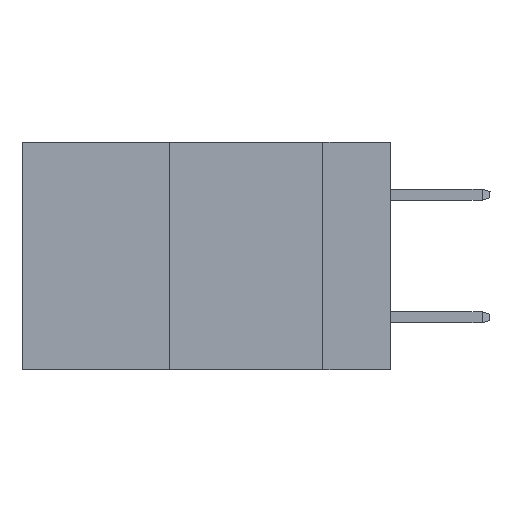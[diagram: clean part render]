
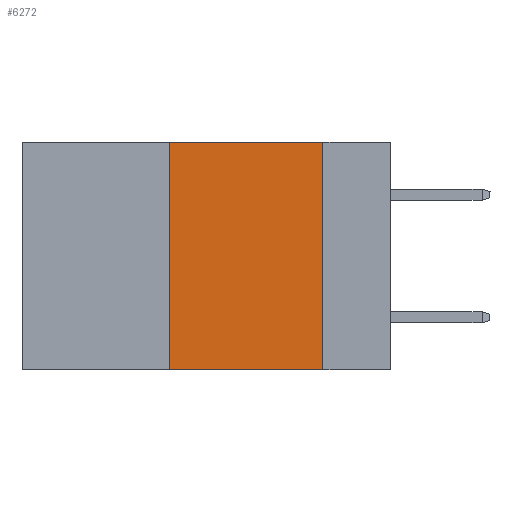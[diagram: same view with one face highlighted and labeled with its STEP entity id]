
A CAD part, left-side view. The second image highlights one B-rep face of the part: STEP entity #6272.
In plain terms, the highlighted planar face has unit normal (-1, 0, 0).
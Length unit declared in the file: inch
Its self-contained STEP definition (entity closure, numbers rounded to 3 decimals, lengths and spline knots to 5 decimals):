
#139 = VERTEX_POINT ( 'NONE', #652 ) ;
#343 = EDGE_LOOP ( 'NONE', ( #1356, #3575, #8555, #2257 ) ) ;
#652 = CARTESIAN_POINT ( 'NONE',  ( 0., 0.11, -0.37 ) ) ;
#679 = EDGE_CURVE ( 'NONE', #9667, #1907, #9324, .T. ) ;
#726 = VECTOR ( 'NONE', #9469, 39.37008 ) ;
#1188 = CARTESIAN_POINT ( 'NONE',  ( 0., 0.36, 0. ) ) ;
#1356 = ORIENTED_EDGE ( 'NONE', *, *, #13403, .F. ) ;
#1403 = VECTOR ( 'NONE', #3296, 39.37008 ) ;
#1476 = VECTOR ( 'NONE', #12735, 39.37008 ) ;
#1731 = LINE ( 'NONE', #4994, #1403 ) ;
#1907 = VERTEX_POINT ( 'NONE', #1188 ) ;
#2257 = ORIENTED_EDGE ( 'NONE', *, *, #3975, .T. ) ;
#3296 = DIRECTION ( 'NONE',  ( 0., -1., 0. ) ) ;
#3575 = ORIENTED_EDGE ( 'NONE', *, *, #12182, .F. ) ;
#3708 = CARTESIAN_POINT ( 'NONE',  ( 0., 0.6, 0. ) ) ;
#3975 = EDGE_CURVE ( 'NONE', #9667, #139, #1731, .T. ) ;
#4302 = CARTESIAN_POINT ( 'NONE',  ( 0., 0.6, 0. ) ) ;
#4690 = LINE ( 'NONE', #4302, #1476 ) ;
#4837 = DIRECTION ( 'NONE',  ( 1., 0., 0. ) ) ;
#4884 = CARTESIAN_POINT ( 'NONE',  ( 0., 0.36, -0.37 ) ) ;
#4994 = CARTESIAN_POINT ( 'NONE',  ( 0., 0.6, -0.37 ) ) ;
#6007 = CARTESIAN_POINT ( 'NONE',  ( 0., 0.11, 0. ) ) ;
#6272 = ADVANCED_FACE ( 'NONE', ( #8806 ), #10167, .F. ) ;
#6329 = AXIS2_PLACEMENT_3D ( 'NONE', #3708, #4837, #12206 ) ;
#7103 = DIRECTION ( 'NONE',  ( 0., 0., -1. ) ) ;
#8555 = ORIENTED_EDGE ( 'NONE', *, *, #679, .F. ) ;
#8806 = FACE_OUTER_BOUND ( 'NONE', #343, .T. ) ;
#9324 = LINE ( 'NONE', #13386, #726 ) ;
#9469 = DIRECTION ( 'NONE',  ( 0., 0., 1. ) ) ;
#9667 = VERTEX_POINT ( 'NONE', #4884 ) ;
#10167 = PLANE ( 'NONE',  #6329 ) ;
#12182 = EDGE_CURVE ( 'NONE', #1907, #12482, #4690, .T. ) ;
#12206 = DIRECTION ( 'NONE',  ( 0., 0., -1. ) ) ;
#12482 = VERTEX_POINT ( 'NONE', #13094 ) ;
#12735 = DIRECTION ( 'NONE',  ( 0., -1., 0. ) ) ;
#13094 = CARTESIAN_POINT ( 'NONE',  ( 0., 0.11, 0. ) ) ;
#13187 = VECTOR ( 'NONE', #7103, 39.37008 ) ;
#13386 = CARTESIAN_POINT ( 'NONE',  ( 0., 0.36, 0. ) ) ;
#13403 = EDGE_CURVE ( 'NONE', #12482, #139, #13489, .T. ) ;
#13489 = LINE ( 'NONE', #6007, #13187 ) ;
